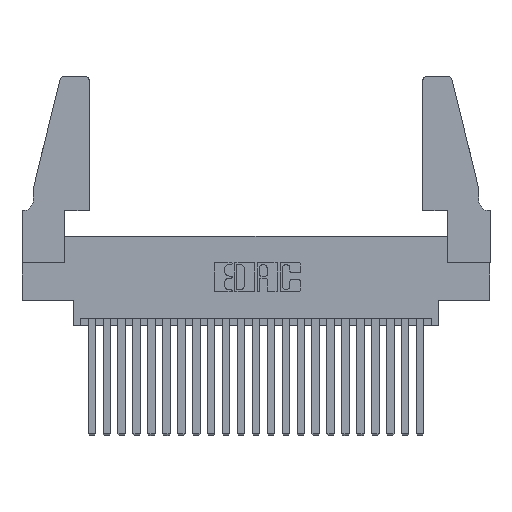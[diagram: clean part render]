
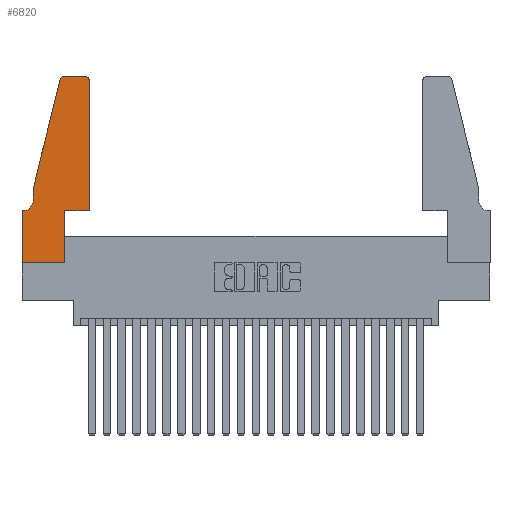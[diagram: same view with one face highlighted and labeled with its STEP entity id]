
A CAD part, top view. The second image highlights one B-rep face of the part: STEP entity #6820.
In plain terms, the highlighted planar face has unit normal (0, 0, 1).
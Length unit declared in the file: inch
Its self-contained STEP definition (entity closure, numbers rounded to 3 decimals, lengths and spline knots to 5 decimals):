
#9 = DIRECTION ( 'NONE',  ( 0., -1., 0. ) ) ;
#274 = CARTESIAN_POINT ( 'NONE',  ( 0.0755, 0.42, 0.37 ) ) ;
#372 = CARTESIAN_POINT ( 'NONE',  ( 0.2865, 0.35, 0.37 ) ) ;
#558 = LINE ( 'NONE', #16955, #14282 ) ;
#726 = EDGE_CURVE ( 'NONE', #21720, #12300, #2779, .T. ) ;
#756 = VECTOR ( 'NONE', #4230, 39.37008 ) ;
#927 = CARTESIAN_POINT ( 'NONE',  ( 0., 0., 0.37 ) ) ;
#1844 = AXIS2_PLACEMENT_3D ( 'NONE', #10740, #22614, #12485 ) ;
#1995 = FACE_OUTER_BOUND ( 'NONE', #3225, .T. ) ;
#2301 = VECTOR ( 'NONE', #15155, 39.37008 ) ;
#2445 = CIRCLE ( 'NONE', #1844, 0.03 ) ;
#2563 = DIRECTION ( 'NONE',  ( 0., 0., -1. ) ) ;
#2652 = CARTESIAN_POINT ( 'NONE',  ( 0.0055, 0.42, 0.37 ) ) ;
#2724 = CARTESIAN_POINT ( 'NONE',  ( 0.4205, 1.25, 0.37 ) ) ;
#2770 = CIRCLE ( 'NONE', #16925, 0.03 ) ;
#2779 = CIRCLE ( 'NONE', #18504, 0.07 ) ;
#2878 = VERTEX_POINT ( 'NONE', #18616 ) ;
#3202 = EDGE_CURVE ( 'NONE', #11487, #19679, #19349, .T. ) ;
#3225 = EDGE_LOOP ( 'NONE', ( #21474, #17989, #3952, #15453, #18613, #15599, #20601, #11867, #5224, #6090, #19534, #8435 ) ) ;
#3394 = CARTESIAN_POINT ( 'NONE',  ( 0.2865, 0.35, 0.37 ) ) ;
#3504 = DIRECTION ( 'NONE',  ( -1., 0., 0. ) ) ;
#3532 = CARTESIAN_POINT ( 'NONE',  ( 0.284, 1.22, 0.37 ) ) ;
#3685 = CARTESIAN_POINT ( 'NONE',  ( 0.0755, 0.5, 0.37 ) ) ;
#3952 = ORIENTED_EDGE ( 'NONE', *, *, #12413, .T. ) ;
#4230 = DIRECTION ( 'NONE',  ( 1., 0., 0. ) ) ;
#5129 = CARTESIAN_POINT ( 'NONE',  ( 0., 0., 0.37 ) ) ;
#5224 = ORIENTED_EDGE ( 'NONE', *, *, #9694, .T. ) ;
#5349 = DIRECTION ( 'NONE',  ( 1., 0., 0. ) ) ;
#5369 = DIRECTION ( 'NONE',  ( 1., 0., 0. ) ) ;
#5685 = DIRECTION ( 'NONE',  ( 0., 1., 0. ) ) ;
#6090 = ORIENTED_EDGE ( 'NONE', *, *, #19938, .T. ) ;
#6304 = LINE ( 'NONE', #3685, #18981 ) ;
#6566 = EDGE_CURVE ( 'NONE', #17760, #2878, #7708, .T. ) ;
#6820 = ADVANCED_FACE ( 'NONE', ( #1995 ), #14140, .T. ) ;
#6908 = VERTEX_POINT ( 'NONE', #21164 ) ;
#6965 = DIRECTION ( 'NONE',  ( 1., 0., 0. ) ) ;
#7120 = VERTEX_POINT ( 'NONE', #11513 ) ;
#7162 = VERTEX_POINT ( 'NONE', #2724 ) ;
#7708 = LINE ( 'NONE', #927, #2301 ) ;
#7902 = AXIS2_PLACEMENT_3D ( 'NONE', #10706, #15806, #5369 ) ;
#7965 = CARTESIAN_POINT ( 'NONE',  ( 0.25487, 1.22718, 0.37 ) ) ;
#8109 = VERTEX_POINT ( 'NONE', #3394 ) ;
#8435 = ORIENTED_EDGE ( 'NONE', *, *, #9451, .T. ) ;
#9418 = CARTESIAN_POINT ( 'NONE',  ( 0.0755, 0.35, 0.37 ) ) ;
#9451 = EDGE_CURVE ( 'NONE', #19679, #7162, #2445, .T. ) ;
#9694 = EDGE_CURVE ( 'NONE', #7120, #8109, #15662, .T. ) ;
#9870 = VECTOR ( 'NONE', #14368, 39.37008 ) ;
#10082 = EDGE_CURVE ( 'NONE', #2878, #7120, #21234, .T. ) ;
#10706 = CARTESIAN_POINT ( 'NONE',  ( 0., 0.35, 0.37 ) ) ;
#10740 = CARTESIAN_POINT ( 'NONE',  ( 0.4205, 1.22, 0.37 ) ) ;
#11169 = VECTOR ( 'NONE', #12975, 39.37008 ) ;
#11487 = VERTEX_POINT ( 'NONE', #16118 ) ;
#11513 = CARTESIAN_POINT ( 'NONE',  ( 0.2865, 0., 0.37 ) ) ;
#11867 = ORIENTED_EDGE ( 'NONE', *, *, #10082, .T. ) ;
#12238 = VECTOR ( 'NONE', #6965, 39.37008 ) ;
#12300 = VERTEX_POINT ( 'NONE', #14969 ) ;
#12413 = EDGE_CURVE ( 'NONE', #16937, #16868, #558, .T. ) ;
#12485 = DIRECTION ( 'NONE',  ( 1., 0., 0. ) ) ;
#12809 = CARTESIAN_POINT ( 'NONE',  ( 0.4505, 0.35, 0.37 ) ) ;
#12975 = DIRECTION ( 'NONE',  ( 0., 1., 0. ) ) ;
#13100 = CARTESIAN_POINT ( 'NONE',  ( 0.4505, 0.35, 0.37 ) ) ;
#13263 = EDGE_CURVE ( 'NONE', #7162, #6908, #14447, .T. ) ;
#13774 = LINE ( 'NONE', #13100, #756 ) ;
#13888 = CARTESIAN_POINT ( 'NONE',  ( 0.4505, 1.22, 0.37 ) ) ;
#14140 = PLANE ( 'NONE',  #7902 ) ;
#14197 = EDGE_CURVE ( 'NONE', #6908, #16937, #2770, .T. ) ;
#14282 = VECTOR ( 'NONE', #20385, 39.37008 ) ;
#14368 = DIRECTION ( 'NONE',  ( -1., 0., 0. ) ) ;
#14447 = LINE ( 'NONE', #19374, #9870 ) ;
#14969 = CARTESIAN_POINT ( 'NONE',  ( 0.0055, 0.35, 0.37 ) ) ;
#15155 = DIRECTION ( 'NONE',  ( 0., -1., 0. ) ) ;
#15453 = ORIENTED_EDGE ( 'NONE', *, *, #17301, .T. ) ;
#15599 = ORIENTED_EDGE ( 'NONE', *, *, #16316, .T. ) ;
#15662 = LINE ( 'NONE', #372, #11169 ) ;
#15787 = DIRECTION ( 'NONE',  ( 0., 0., 1. ) ) ;
#15806 = DIRECTION ( 'NONE',  ( 0., 0., 1. ) ) ;
#16118 = CARTESIAN_POINT ( 'NONE',  ( 0.4505, 0.35, 0.37 ) ) ;
#16316 = EDGE_CURVE ( 'NONE', #12300, #17760, #17717, .T. ) ;
#16868 = VERTEX_POINT ( 'NONE', #18028 ) ;
#16925 = AXIS2_PLACEMENT_3D ( 'NONE', #3532, #15787, #5349 ) ;
#16937 = VERTEX_POINT ( 'NONE', #7965 ) ;
#16955 = CARTESIAN_POINT ( 'NONE',  ( 0.0755, 0.5, 0.37 ) ) ;
#17182 = VECTOR ( 'NONE', #21371, 39.37008 ) ;
#17301 = EDGE_CURVE ( 'NONE', #16868, #21720, #6304, .T. ) ;
#17717 = LINE ( 'NONE', #9418, #17182 ) ;
#17760 = VERTEX_POINT ( 'NONE', #19099 ) ;
#17989 = ORIENTED_EDGE ( 'NONE', *, *, #14197, .T. ) ;
#18028 = CARTESIAN_POINT ( 'NONE',  ( 0.0755, 0.5, 0.37 ) ) ;
#18504 = AXIS2_PLACEMENT_3D ( 'NONE', #2652, #2563, #3504 ) ;
#18613 = ORIENTED_EDGE ( 'NONE', *, *, #726, .T. ) ;
#18616 = CARTESIAN_POINT ( 'NONE',  ( 0., 0., 0.37 ) ) ;
#18799 = VECTOR ( 'NONE', #5685, 39.37008 ) ;
#18981 = VECTOR ( 'NONE', #9, 39.37008 ) ;
#19099 = CARTESIAN_POINT ( 'NONE',  ( 0., 0.35, 0.37 ) ) ;
#19349 = LINE ( 'NONE', #12809, #18799 ) ;
#19374 = CARTESIAN_POINT ( 'NONE',  ( 0.2605, 1.25, 0.37 ) ) ;
#19534 = ORIENTED_EDGE ( 'NONE', *, *, #3202, .T. ) ;
#19679 = VERTEX_POINT ( 'NONE', #13888 ) ;
#19938 = EDGE_CURVE ( 'NONE', #8109, #11487, #13774, .T. ) ;
#20385 = DIRECTION ( 'NONE',  ( -0.239, -0.971, 0. ) ) ;
#20601 = ORIENTED_EDGE ( 'NONE', *, *, #6566, .T. ) ;
#21164 = CARTESIAN_POINT ( 'NONE',  ( 0.284, 1.25, 0.37 ) ) ;
#21234 = LINE ( 'NONE', #5129, #12238 ) ;
#21371 = DIRECTION ( 'NONE',  ( -1., 0., 0. ) ) ;
#21474 = ORIENTED_EDGE ( 'NONE', *, *, #13263, .T. ) ;
#21720 = VERTEX_POINT ( 'NONE', #274 ) ;
#22614 = DIRECTION ( 'NONE',  ( 0., 0., 1. ) ) ;
